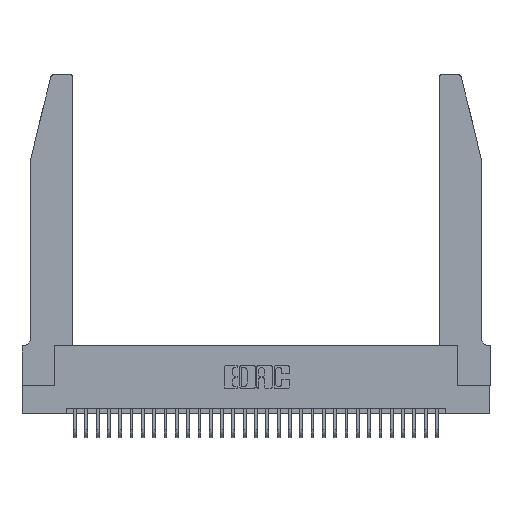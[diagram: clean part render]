
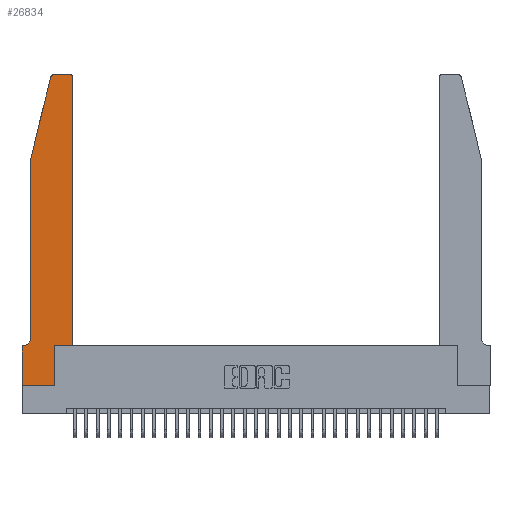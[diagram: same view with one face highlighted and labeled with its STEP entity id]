
A CAD part, top view. The second image highlights one B-rep face of the part: STEP entity #26834.
In plain terms, the highlighted planar face has unit normal (0, 0, 1).
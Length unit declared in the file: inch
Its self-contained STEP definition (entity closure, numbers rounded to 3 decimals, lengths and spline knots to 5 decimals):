
#658 = CARTESIAN_POINT ( 'NONE',  ( 0.284, 2.72, 0.37 ) ) ;
#1033 = PLANE ( 'NONE',  #25072 ) ;
#1040 = VERTEX_POINT ( 'NONE', #15308 ) ;
#1370 = EDGE_CURVE ( 'NONE', #11045, #8528, #14312, .T. ) ;
#1466 = ORIENTED_EDGE ( 'NONE', *, *, #19652, .T. ) ;
#1615 = VECTOR ( 'NONE', #30289, 39.37008 ) ;
#1725 = CARTESIAN_POINT ( 'NONE',  ( 0.0755, 0.42, 0.37 ) ) ;
#2336 = DIRECTION ( 'NONE',  ( 0., 0., 1. ) ) ;
#2883 = CARTESIAN_POINT ( 'NONE',  ( 0., 0., 0.37 ) ) ;
#3441 = EDGE_CURVE ( 'NONE', #1040, #16948, #7752, .T. ) ;
#3973 = ORIENTED_EDGE ( 'NONE', *, *, #3441, .T. ) ;
#4080 = VECTOR ( 'NONE', #23608, 39.37008 ) ;
#4146 = DIRECTION ( 'NONE',  ( 0., 1., 0. ) ) ;
#4306 = CARTESIAN_POINT ( 'NONE',  ( 0.284, 2.75, 0.37 ) ) ;
#4659 = EDGE_CURVE ( 'NONE', #10401, #21520, #14952, .T. ) ;
#5668 = LINE ( 'NONE', #19602, #20229 ) ;
#5695 = DIRECTION ( 'NONE',  ( 0., 1., 0. ) ) ;
#5937 = VECTOR ( 'NONE', #16309, 39.37008 ) ;
#6030 = EDGE_CURVE ( 'NONE', #18855, #1040, #13642, .T. ) ;
#6891 = ORIENTED_EDGE ( 'NONE', *, *, #11950, .T. ) ;
#6981 = ORIENTED_EDGE ( 'NONE', *, *, #21705, .T. ) ;
#7490 = CARTESIAN_POINT ( 'NONE',  ( 0.4505, 2.72, 0.37 ) ) ;
#7752 = LINE ( 'NONE', #33077, #17066 ) ;
#8122 = ORIENTED_EDGE ( 'NONE', *, *, #31790, .T. ) ;
#8528 = VERTEX_POINT ( 'NONE', #19639 ) ;
#8910 = AXIS2_PLACEMENT_3D ( 'NONE', #658, #26457, #23528 ) ;
#9208 = DIRECTION ( 'NONE',  ( 0., 0., 1. ) ) ;
#9220 = VECTOR ( 'NONE', #4146, 39.37008 ) ;
#9455 = DIRECTION ( 'NONE',  ( -1., 0., 0. ) ) ;
#9738 = CARTESIAN_POINT ( 'NONE',  ( 0., 0.35, 0.37 ) ) ;
#10401 = VERTEX_POINT ( 'NONE', #7490 ) ;
#10405 = LINE ( 'NONE', #15999, #21715 ) ;
#11045 = VERTEX_POINT ( 'NONE', #15307 ) ;
#11136 = CARTESIAN_POINT ( 'NONE',  ( 0.0055, 0.42, 0.37 ) ) ;
#11803 = VECTOR ( 'NONE', #14955, 39.37008 ) ;
#11950 = EDGE_CURVE ( 'NONE', #16948, #10401, #10405, .T. ) ;
#12086 = CARTESIAN_POINT ( 'NONE',  ( 0.2605, 2.75, 0.37 ) ) ;
#12482 = CIRCLE ( 'NONE', #29926, 0.07 ) ;
#13547 = ORIENTED_EDGE ( 'NONE', *, *, #6030, .T. ) ;
#13642 = LINE ( 'NONE', #26119, #9220 ) ;
#14274 = DIRECTION ( 'NONE',  ( 1., 0., 0. ) ) ;
#14312 = LINE ( 'NONE', #22637, #30073 ) ;
#14397 = EDGE_CURVE ( 'NONE', #8528, #17103, #20498, .T. ) ;
#14747 = VERTEX_POINT ( 'NONE', #9738 ) ;
#14817 = CARTESIAN_POINT ( 'NONE',  ( 0.4205, 2.72, 0.37 ) ) ;
#14952 = CIRCLE ( 'NONE', #24634, 0.03 ) ;
#14955 = DIRECTION ( 'NONE',  ( 0., -1., 0. ) ) ;
#15307 = CARTESIAN_POINT ( 'NONE',  ( 0.25487, 2.72718, 0.37 ) ) ;
#15308 = CARTESIAN_POINT ( 'NONE',  ( 0.2865, 0.35, 0.37 ) ) ;
#15999 = CARTESIAN_POINT ( 'NONE',  ( 0.4505, 0.35, 0.37 ) ) ;
#16309 = DIRECTION ( 'NONE',  ( 0., -1., 0. ) ) ;
#16886 = CARTESIAN_POINT ( 'NONE',  ( 0., 0.35, 0.37 ) ) ;
#16948 = VERTEX_POINT ( 'NONE', #32372 ) ;
#17066 = VECTOR ( 'NONE', #22687, 39.37008 ) ;
#17103 = VERTEX_POINT ( 'NONE', #1725 ) ;
#17449 = CARTESIAN_POINT ( 'NONE',  ( 0., 0., 0.37 ) ) ;
#18176 = FACE_OUTER_BOUND ( 'NONE', #23470, .T. ) ;
#18184 = ORIENTED_EDGE ( 'NONE', *, *, #14397, .T. ) ;
#18633 = CARTESIAN_POINT ( 'NONE',  ( 0., 0., 0.37 ) ) ;
#18670 = ORIENTED_EDGE ( 'NONE', *, *, #1370, .T. ) ;
#18855 = VERTEX_POINT ( 'NONE', #28208 ) ;
#18928 = DIRECTION ( 'NONE',  ( -1., 0., 0. ) ) ;
#19602 = CARTESIAN_POINT ( 'NONE',  ( 0.0755, 0.35, 0.37 ) ) ;
#19639 = CARTESIAN_POINT ( 'NONE',  ( 0.0755, 2., 0.37 ) ) ;
#19652 = EDGE_CURVE ( 'NONE', #30850, #11045, #29455, .T. ) ;
#19977 = EDGE_CURVE ( 'NONE', #26403, #14747, #5668, .T. ) ;
#20229 = VECTOR ( 'NONE', #9455, 39.37008 ) ;
#20498 = LINE ( 'NONE', #21277, #5937 ) ;
#20967 = ORIENTED_EDGE ( 'NONE', *, *, #32691, .T. ) ;
#21095 = VERTEX_POINT ( 'NONE', #18633 ) ;
#21272 = DIRECTION ( 'NONE',  ( -0.239, -0.971, 0. ) ) ;
#21277 = CARTESIAN_POINT ( 'NONE',  ( 0.0755, 2., 0.37 ) ) ;
#21520 = VERTEX_POINT ( 'NONE', #30603 ) ;
#21705 = EDGE_CURVE ( 'NONE', #17103, #26403, #12482, .T. ) ;
#21715 = VECTOR ( 'NONE', #5695, 39.37008 ) ;
#22267 = LINE ( 'NONE', #12086, #1615 ) ;
#22298 = LINE ( 'NONE', #2883, #4080 ) ;
#22340 = CARTESIAN_POINT ( 'NONE',  ( 0.0055, 0.35, 0.37 ) ) ;
#22637 = CARTESIAN_POINT ( 'NONE',  ( 0.0755, 2., 0.37 ) ) ;
#22687 = DIRECTION ( 'NONE',  ( 1., 0., 0. ) ) ;
#22878 = ORIENTED_EDGE ( 'NONE', *, *, #19977, .T. ) ;
#22911 = ORIENTED_EDGE ( 'NONE', *, *, #4659, .T. ) ;
#23068 = DIRECTION ( 'NONE',  ( 1., 0., 0. ) ) ;
#23470 = EDGE_LOOP ( 'NONE', ( #20967, #1466, #18670, #18184, #6981, #22878, #31268, #8122, #13547, #3973, #6891, #22911 ) ) ;
#23528 = DIRECTION ( 'NONE',  ( 1., 0., 0. ) ) ;
#23608 = DIRECTION ( 'NONE',  ( 1., 0., 0. ) ) ;
#24634 = AXIS2_PLACEMENT_3D ( 'NONE', #14817, #2336, #23068 ) ;
#25072 = AXIS2_PLACEMENT_3D ( 'NONE', #16886, #9208, #14274 ) ;
#25163 = LINE ( 'NONE', #17449, #11803 ) ;
#26119 = CARTESIAN_POINT ( 'NONE',  ( 0.2865, 0.35, 0.37 ) ) ;
#26403 = VERTEX_POINT ( 'NONE', #22340 ) ;
#26457 = DIRECTION ( 'NONE',  ( 0., 0., 1. ) ) ;
#26834 = ADVANCED_FACE ( 'NONE', ( #18176 ), #1033, .T. ) ;
#28208 = CARTESIAN_POINT ( 'NONE',  ( 0.2865, 0., 0.37 ) ) ;
#29455 = CIRCLE ( 'NONE', #8910, 0.03 ) ;
#29926 = AXIS2_PLACEMENT_3D ( 'NONE', #11136, #32047, #18928 ) ;
#30073 = VECTOR ( 'NONE', #21272, 39.37008 ) ;
#30289 = DIRECTION ( 'NONE',  ( -1., 0., 0. ) ) ;
#30603 = CARTESIAN_POINT ( 'NONE',  ( 0.4205, 2.75, 0.37 ) ) ;
#30761 = EDGE_CURVE ( 'NONE', #14747, #21095, #25163, .T. ) ;
#30850 = VERTEX_POINT ( 'NONE', #4306 ) ;
#31268 = ORIENTED_EDGE ( 'NONE', *, *, #30761, .T. ) ;
#31790 = EDGE_CURVE ( 'NONE', #21095, #18855, #22298, .T. ) ;
#32047 = DIRECTION ( 'NONE',  ( 0., 0., -1. ) ) ;
#32372 = CARTESIAN_POINT ( 'NONE',  ( 0.4505, 0.35, 0.37 ) ) ;
#32691 = EDGE_CURVE ( 'NONE', #21520, #30850, #22267, .T. ) ;
#33077 = CARTESIAN_POINT ( 'NONE',  ( 0.4505, 0.35, 0.37 ) ) ;
